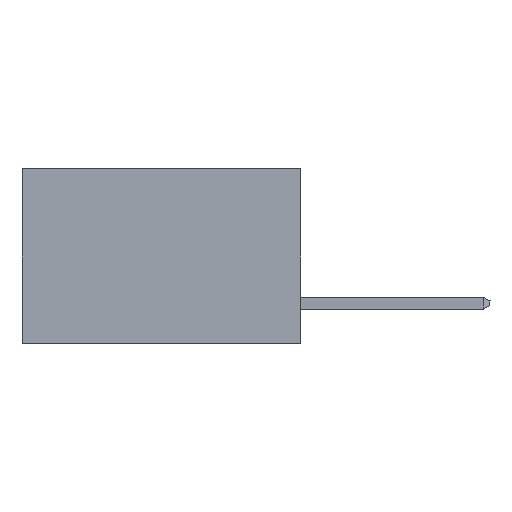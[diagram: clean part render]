
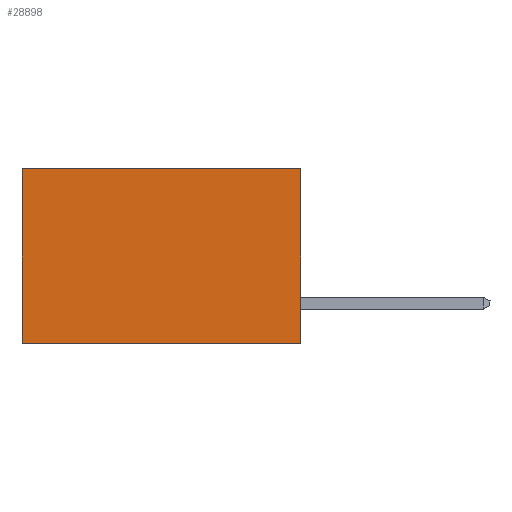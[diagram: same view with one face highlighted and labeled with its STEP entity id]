
A CAD part, left-side view. The second image highlights one B-rep face of the part: STEP entity #28898.
In plain terms, the highlighted planar face has unit normal (-1, 0, 0).
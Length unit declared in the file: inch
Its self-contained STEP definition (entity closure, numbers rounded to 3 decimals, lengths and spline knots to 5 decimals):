
#815 = CARTESIAN_POINT ( 'NONE',  ( 0.277, 0., 0. ) ) ;
#1026 = EDGE_CURVE ( 'NONE', #4527, #26258, #1386, .T. ) ;
#1118 = FACE_OUTER_BOUND ( 'NONE', #8150, .T. ) ;
#1249 = ORIENTED_EDGE ( 'NONE', *, *, #2469, .T. ) ;
#1386 = LINE ( 'NONE', #14275, #7116 ) ;
#2233 = EDGE_CURVE ( 'NONE', #9909, #4527, #29844, .T. ) ;
#2469 = EDGE_CURVE ( 'NONE', #2538, #26258, #28737, .T. ) ;
#2538 = VERTEX_POINT ( 'NONE', #21695 ) ;
#4527 = VERTEX_POINT ( 'NONE', #14000 ) ;
#6285 = CARTESIAN_POINT ( 'NONE',  ( 0.277, 0.59, -0.37 ) ) ;
#6863 = VECTOR ( 'NONE', #25036, 39.37008 ) ;
#7116 = VECTOR ( 'NONE', #27912, 39.37008 ) ;
#8009 = ORIENTED_EDGE ( 'NONE', *, *, #16252, .T. ) ;
#8150 = EDGE_LOOP ( 'NONE', ( #1249, #24317, #29741, #8009 ) ) ;
#8803 = PLANE ( 'NONE',  #23214 ) ;
#9909 = VERTEX_POINT ( 'NONE', #26789 ) ;
#13339 = LINE ( 'NONE', #815, #6863 ) ;
#13661 = DIRECTION ( 'NONE',  ( 1., 0., 0. ) ) ;
#14000 = CARTESIAN_POINT ( 'NONE',  ( 0.277, 0., -0.37 ) ) ;
#14275 = CARTESIAN_POINT ( 'NONE',  ( 0.277, 0., -0.37 ) ) ;
#15815 = CARTESIAN_POINT ( 'NONE',  ( 0.277, 0., -0.37 ) ) ;
#16252 = EDGE_CURVE ( 'NONE', #9909, #2538, #13339, .T. ) ;
#16915 = VECTOR ( 'NONE', #26793, 39.37008 ) ;
#17758 = DIRECTION ( 'NONE',  ( 0., 0., -1. ) ) ;
#21695 = CARTESIAN_POINT ( 'NONE',  ( 0.277, 0.59, 0. ) ) ;
#23214 = AXIS2_PLACEMENT_3D ( 'NONE', #27959, #13661, #30261 ) ;
#23675 = VECTOR ( 'NONE', #17758, 39.37008 ) ;
#24317 = ORIENTED_EDGE ( 'NONE', *, *, #1026, .F. ) ;
#24960 = CARTESIAN_POINT ( 'NONE',  ( 0.277, 0.59, -0.37 ) ) ;
#25036 = DIRECTION ( 'NONE',  ( 0., 1., 0. ) ) ;
#26258 = VERTEX_POINT ( 'NONE', #6285 ) ;
#26789 = CARTESIAN_POINT ( 'NONE',  ( 0.277, 0., 0. ) ) ;
#26793 = DIRECTION ( 'NONE',  ( 0., 0., -1. ) ) ;
#27912 = DIRECTION ( 'NONE',  ( 0., 1., 0. ) ) ;
#27959 = CARTESIAN_POINT ( 'NONE',  ( 0.277, 0., -0.37 ) ) ;
#28737 = LINE ( 'NONE', #24960, #16915 ) ;
#28898 = ADVANCED_FACE ( 'NONE', ( #1118 ), #8803, .F. ) ;
#29741 = ORIENTED_EDGE ( 'NONE', *, *, #2233, .F. ) ;
#29844 = LINE ( 'NONE', #15815, #23675 ) ;
#30261 = DIRECTION ( 'NONE',  ( 0., 0., -1. ) ) ;
